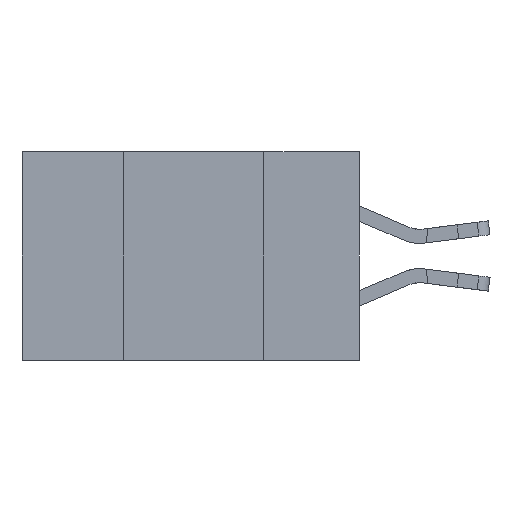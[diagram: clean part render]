
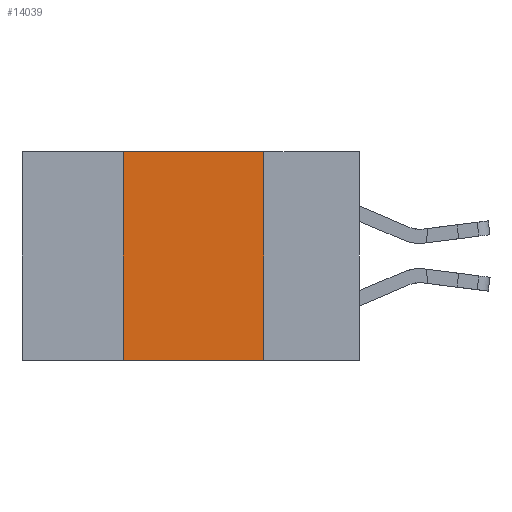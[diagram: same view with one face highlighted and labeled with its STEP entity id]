
A CAD part, left-side view. The second image highlights one B-rep face of the part: STEP entity #14039.
In plain terms, the highlighted planar face has unit normal (-1, 0, 0).
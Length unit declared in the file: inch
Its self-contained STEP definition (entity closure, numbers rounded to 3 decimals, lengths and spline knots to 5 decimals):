
#1192 = DIRECTION ( 'NONE',  ( 0., 0., -1. ) ) ;
#1986 = VECTOR ( 'NONE', #2826, 39.37008 ) ;
#2246 = DIRECTION ( 'NONE',  ( 1., 0., 0. ) ) ;
#2826 = DIRECTION ( 'NONE',  ( 0., -1., 0. ) ) ;
#3608 = CARTESIAN_POINT ( 'NONE',  ( 0., 0.17, 0. ) ) ;
#4230 = CARTESIAN_POINT ( 'NONE',  ( 0., 0.42, -0.37 ) ) ;
#4409 = CARTESIAN_POINT ( 'NONE',  ( 0., 0.6, -0.37 ) ) ;
#4943 = VERTEX_POINT ( 'NONE', #3608 ) ;
#5047 = EDGE_CURVE ( 'NONE', #17073, #13418, #16526, .T. ) ;
#6919 = ORIENTED_EDGE ( 'NONE', *, *, #16281, .F. ) ;
#7433 = DIRECTION ( 'NONE',  ( 0., -1., 0. ) ) ;
#7767 = VERTEX_POINT ( 'NONE', #17617 ) ;
#8936 = VECTOR ( 'NONE', #7433, 39.37008 ) ;
#9000 = CARTESIAN_POINT ( 'NONE',  ( 0., 0.42, 0. ) ) ;
#9001 = ORIENTED_EDGE ( 'NONE', *, *, #15516, .F. ) ;
#9434 = LINE ( 'NONE', #18852, #8936 ) ;
#10357 = CARTESIAN_POINT ( 'NONE',  ( 0., 0.6, 0. ) ) ;
#11582 = ORIENTED_EDGE ( 'NONE', *, *, #5047, .F. ) ;
#11660 = VECTOR ( 'NONE', #16913, 39.37008 ) ;
#13008 = LINE ( 'NONE', #19093, #16330 ) ;
#13418 = VERTEX_POINT ( 'NONE', #9000 ) ;
#13533 = EDGE_LOOP ( 'NONE', ( #6919, #9001, #11582, #20192 ) ) ;
#13623 = DIRECTION ( 'NONE',  ( 0., 0., -1. ) ) ;
#13687 = FACE_OUTER_BOUND ( 'NONE', #13533, .T. ) ;
#13754 = EDGE_CURVE ( 'NONE', #17073, #7767, #19297, .T. ) ;
#14039 = ADVANCED_FACE ( 'NONE', ( #13687 ), #16858, .F. ) ;
#15247 = CARTESIAN_POINT ( 'NONE',  ( 0., 0.42, 0. ) ) ;
#15516 = EDGE_CURVE ( 'NONE', #13418, #4943, #9434, .T. ) ;
#16281 = EDGE_CURVE ( 'NONE', #4943, #7767, #13008, .T. ) ;
#16330 = VECTOR ( 'NONE', #1192, 39.37008 ) ;
#16526 = LINE ( 'NONE', #15247, #11660 ) ;
#16858 = PLANE ( 'NONE',  #16958 ) ;
#16913 = DIRECTION ( 'NONE',  ( 0., 0., 1. ) ) ;
#16958 = AXIS2_PLACEMENT_3D ( 'NONE', #10357, #2246, #13623 ) ;
#17073 = VERTEX_POINT ( 'NONE', #4230 ) ;
#17617 = CARTESIAN_POINT ( 'NONE',  ( 0., 0.17, -0.37 ) ) ;
#18852 = CARTESIAN_POINT ( 'NONE',  ( 0., 0.6, 0. ) ) ;
#19093 = CARTESIAN_POINT ( 'NONE',  ( 0., 0.17, 0. ) ) ;
#19297 = LINE ( 'NONE', #4409, #1986 ) ;
#20192 = ORIENTED_EDGE ( 'NONE', *, *, #13754, .T. ) ;
